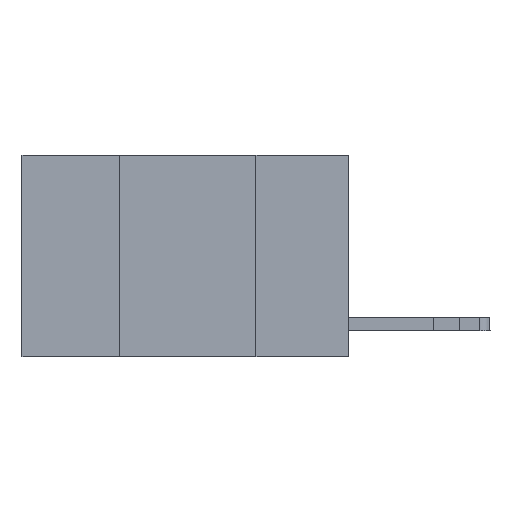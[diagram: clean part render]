
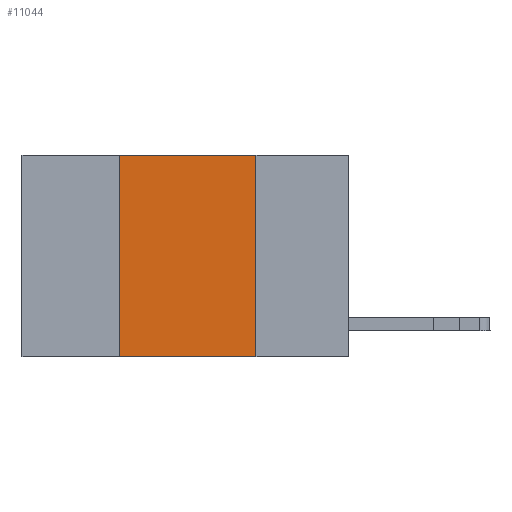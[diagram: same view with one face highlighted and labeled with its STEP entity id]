
A CAD part, left-side view. The second image highlights one B-rep face of the part: STEP entity #11044.
In plain terms, the highlighted planar face has unit normal (-1, 0, 0).
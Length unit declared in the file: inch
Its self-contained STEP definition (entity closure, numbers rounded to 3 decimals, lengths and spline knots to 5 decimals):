
#486 = ORIENTED_EDGE ( 'NONE', *, *, #14122, .F. ) ;
#1683 = EDGE_CURVE ( 'NONE', #12266, #15140, #12102, .T. ) ;
#2791 = ORIENTED_EDGE ( 'NONE', *, *, #15607, .F. ) ;
#3525 = DIRECTION ( 'NONE',  ( 0., -1., 0. ) ) ;
#4406 = CARTESIAN_POINT ( 'NONE',  ( 0., 0.17, 0. ) ) ;
#5390 = CARTESIAN_POINT ( 'NONE',  ( 0., 0.6, 0. ) ) ;
#6009 = VERTEX_POINT ( 'NONE', #18804 ) ;
#6915 = VERTEX_POINT ( 'NONE', #13132 ) ;
#7053 = DIRECTION ( 'NONE',  ( 0., 0., -1. ) ) ;
#8615 = DIRECTION ( 'NONE',  ( 1., 0., 0. ) ) ;
#9351 = VECTOR ( 'NONE', #15690, 39.37008 ) ;
#10641 = CARTESIAN_POINT ( 'NONE',  ( 0., 0.6, 0. ) ) ;
#11044 = ADVANCED_FACE ( 'NONE', ( #12085 ), #20818, .F. ) ;
#12085 = FACE_OUTER_BOUND ( 'NONE', #16755, .T. ) ;
#12102 = LINE ( 'NONE', #17248, #21644 ) ;
#12266 = VERTEX_POINT ( 'NONE', #4406 ) ;
#12398 = VECTOR ( 'NONE', #3525, 39.37008 ) ;
#12567 = VECTOR ( 'NONE', #15050, 39.37008 ) ;
#12860 = AXIS2_PLACEMENT_3D ( 'NONE', #10641, #8615, #7053 ) ;
#13132 = CARTESIAN_POINT ( 'NONE',  ( 0., 0.42, -0.37 ) ) ;
#13715 = LINE ( 'NONE', #18856, #12398 ) ;
#13902 = LINE ( 'NONE', #5390, #9351 ) ;
#14122 = EDGE_CURVE ( 'NONE', #6009, #12266, #13902, .T. ) ;
#15050 = DIRECTION ( 'NONE',  ( 0., 0., 1. ) ) ;
#15140 = VERTEX_POINT ( 'NONE', #21816 ) ;
#15607 = EDGE_CURVE ( 'NONE', #6915, #6009, #18604, .T. ) ;
#15690 = DIRECTION ( 'NONE',  ( 0., -1., 0. ) ) ;
#16755 = EDGE_LOOP ( 'NONE', ( #20652, #486, #2791, #21368 ) ) ;
#17178 = EDGE_CURVE ( 'NONE', #6915, #15140, #13715, .T. ) ;
#17248 = CARTESIAN_POINT ( 'NONE',  ( 0., 0.17, 0. ) ) ;
#17363 = DIRECTION ( 'NONE',  ( 0., 0., -1. ) ) ;
#18494 = CARTESIAN_POINT ( 'NONE',  ( 0., 0.42, 0. ) ) ;
#18604 = LINE ( 'NONE', #18494, #12567 ) ;
#18804 = CARTESIAN_POINT ( 'NONE',  ( 0., 0.42, 0. ) ) ;
#18856 = CARTESIAN_POINT ( 'NONE',  ( 0., 0.6, -0.37 ) ) ;
#20652 = ORIENTED_EDGE ( 'NONE', *, *, #1683, .F. ) ;
#20818 = PLANE ( 'NONE',  #12860 ) ;
#21368 = ORIENTED_EDGE ( 'NONE', *, *, #17178, .T. ) ;
#21644 = VECTOR ( 'NONE', #17363, 39.37008 ) ;
#21816 = CARTESIAN_POINT ( 'NONE',  ( 0., 0.17, -0.37 ) ) ;
